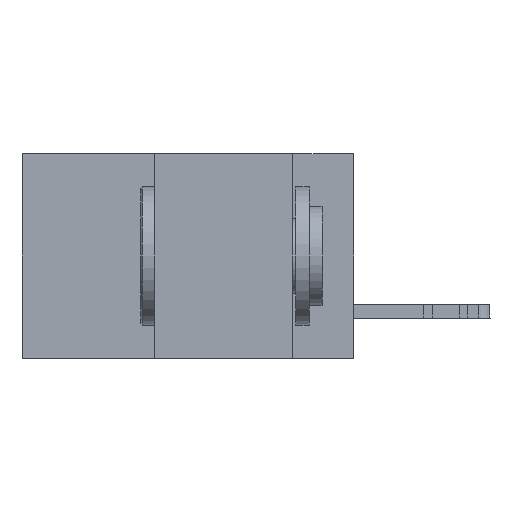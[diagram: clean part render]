
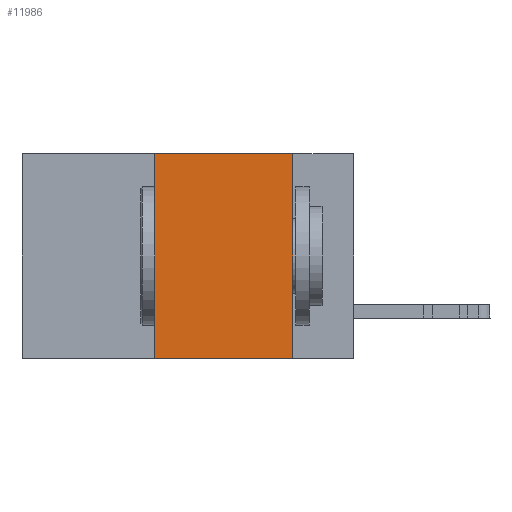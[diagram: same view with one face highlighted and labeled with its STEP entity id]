
A CAD part, left-side view. The second image highlights one B-rep face of the part: STEP entity #11986.
In plain terms, the highlighted planar face has unit normal (-1, 0, 0).
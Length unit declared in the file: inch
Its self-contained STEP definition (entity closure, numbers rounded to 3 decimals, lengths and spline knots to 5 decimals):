
#1417 = CARTESIAN_POINT ( 'NONE',  ( 0., 0.36, 0. ) ) ;
#2700 = VECTOR ( 'NONE', #29919, 39.37008 ) ;
#5013 = LINE ( 'NONE', #20901, #44117 ) ;
#5194 = DIRECTION ( 'NONE',  ( 0., 0., -1. ) ) ;
#6800 = CARTESIAN_POINT ( 'NONE',  ( 0., 0.11, -0.37 ) ) ;
#7889 = CARTESIAN_POINT ( 'NONE',  ( 0., 0.6, 0. ) ) ;
#8041 = AXIS2_PLACEMENT_3D ( 'NONE', #7889, #15112, #18943 ) ;
#8377 = VERTEX_POINT ( 'NONE', #6800 ) ;
#9177 = CARTESIAN_POINT ( 'NONE',  ( 0., 0.11, 0. ) ) ;
#10410 = LINE ( 'NONE', #35023, #48917 ) ;
#10902 = VERTEX_POINT ( 'NONE', #1417 ) ;
#11986 = ADVANCED_FACE ( 'NONE', ( #24915 ), #37824, .F. ) ;
#12298 = ORIENTED_EDGE ( 'NONE', *, *, #14107, .F. ) ;
#13235 = EDGE_CURVE ( 'NONE', #30216, #8377, #32410, .T. ) ;
#14107 = EDGE_CURVE ( 'NONE', #10902, #23995, #16760, .T. ) ;
#15112 = DIRECTION ( 'NONE',  ( 1., 0., 0. ) ) ;
#16760 = LINE ( 'NONE', #48722, #2700 ) ;
#17480 = EDGE_LOOP ( 'NONE', ( #32814, #12298, #34815, #43592 ) ) ;
#18943 = DIRECTION ( 'NONE',  ( 0., 0., -1. ) ) ;
#20901 = CARTESIAN_POINT ( 'NONE',  ( 0., 0.11, 0. ) ) ;
#23995 = VERTEX_POINT ( 'NONE', #9177 ) ;
#24915 = FACE_OUTER_BOUND ( 'NONE', #17480, .T. ) ;
#25157 = CARTESIAN_POINT ( 'NONE',  ( 0., 0.36, -0.37 ) ) ;
#28321 = DIRECTION ( 'NONE',  ( 0., -1., 0. ) ) ;
#29919 = DIRECTION ( 'NONE',  ( 0., -1., 0. ) ) ;
#30216 = VERTEX_POINT ( 'NONE', #25157 ) ;
#32410 = LINE ( 'NONE', #47103, #45353 ) ;
#32814 = ORIENTED_EDGE ( 'NONE', *, *, #38022, .F. ) ;
#34815 = ORIENTED_EDGE ( 'NONE', *, *, #45692, .F. ) ;
#35023 = CARTESIAN_POINT ( 'NONE',  ( 0., 0.36, 0. ) ) ;
#37824 = PLANE ( 'NONE',  #8041 ) ;
#38022 = EDGE_CURVE ( 'NONE', #23995, #8377, #5013, .T. ) ;
#38336 = DIRECTION ( 'NONE',  ( 0., 0., 1. ) ) ;
#43592 = ORIENTED_EDGE ( 'NONE', *, *, #13235, .T. ) ;
#44117 = VECTOR ( 'NONE', #5194, 39.37008 ) ;
#45353 = VECTOR ( 'NONE', #28321, 39.37008 ) ;
#45692 = EDGE_CURVE ( 'NONE', #30216, #10902, #10410, .T. ) ;
#47103 = CARTESIAN_POINT ( 'NONE',  ( 0., 0.6, -0.37 ) ) ;
#48722 = CARTESIAN_POINT ( 'NONE',  ( 0., 0.6, 0. ) ) ;
#48917 = VECTOR ( 'NONE', #38336, 39.37008 ) ;
